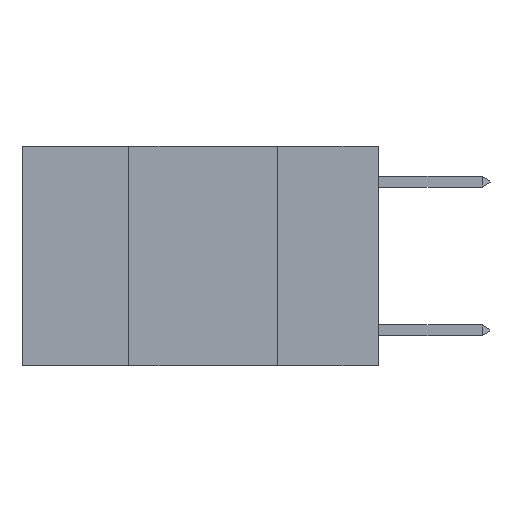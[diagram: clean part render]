
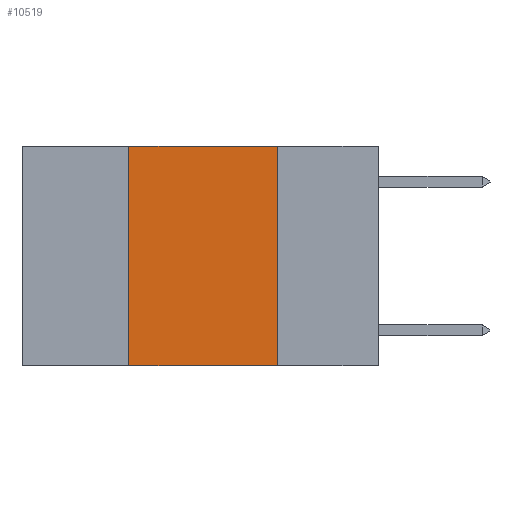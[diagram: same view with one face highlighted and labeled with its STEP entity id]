
A CAD part, left-side view. The second image highlights one B-rep face of the part: STEP entity #10519.
In plain terms, the highlighted planar face has unit normal (-1, 0, 0).
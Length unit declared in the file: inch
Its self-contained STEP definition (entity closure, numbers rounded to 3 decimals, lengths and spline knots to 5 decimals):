
#997 = EDGE_LOOP ( 'NONE', ( #5520, #3920, #13451, #10534 ) ) ;
#1403 = VECTOR ( 'NONE', #11134, 39.37008 ) ;
#1593 = LINE ( 'NONE', #3364, #11028 ) ;
#1623 = DIRECTION ( 'NONE',  ( 0., -1., 0. ) ) ;
#1652 = VECTOR ( 'NONE', #1623, 39.37008 ) ;
#2598 = CARTESIAN_POINT ( 'NONE',  ( 0., 0.17, 0. ) ) ;
#2888 = PLANE ( 'NONE',  #7925 ) ;
#3308 = CARTESIAN_POINT ( 'NONE',  ( 0., 0.17, 0. ) ) ;
#3364 = CARTESIAN_POINT ( 'NONE',  ( 0., 0.42, 0. ) ) ;
#3370 = VECTOR ( 'NONE', #3616, 39.37008 ) ;
#3616 = DIRECTION ( 'NONE',  ( 0., -1., 0. ) ) ;
#3920 = ORIENTED_EDGE ( 'NONE', *, *, #4341, .F. ) ;
#3985 = FACE_OUTER_BOUND ( 'NONE', #997, .T. ) ;
#4327 = VERTEX_POINT ( 'NONE', #8125 ) ;
#4341 = EDGE_CURVE ( 'NONE', #4327, #14167, #11317, .T. ) ;
#4520 = EDGE_CURVE ( 'NONE', #12907, #4327, #1593, .T. ) ;
#5520 = ORIENTED_EDGE ( 'NONE', *, *, #13790, .F. ) ;
#5553 = CARTESIAN_POINT ( 'NONE',  ( 0., 0.17, -0.37 ) ) ;
#7282 = CARTESIAN_POINT ( 'NONE',  ( 0., 0.6, -0.37 ) ) ;
#7313 = CARTESIAN_POINT ( 'NONE',  ( 0., 0.6, 0. ) ) ;
#7388 = CARTESIAN_POINT ( 'NONE',  ( 0., 0.42, -0.37 ) ) ;
#7925 = AXIS2_PLACEMENT_3D ( 'NONE', #7313, #11747, #8471 ) ;
#8125 = CARTESIAN_POINT ( 'NONE',  ( 0., 0.42, 0. ) ) ;
#8471 = DIRECTION ( 'NONE',  ( 0., 0., -1. ) ) ;
#9482 = DIRECTION ( 'NONE',  ( 0., 0., 1. ) ) ;
#10519 = ADVANCED_FACE ( 'NONE', ( #3985 ), #2888, .F. ) ;
#10534 = ORIENTED_EDGE ( 'NONE', *, *, #13945, .T. ) ;
#11028 = VECTOR ( 'NONE', #9482, 39.37008 ) ;
#11134 = DIRECTION ( 'NONE',  ( 0., 0., -1. ) ) ;
#11317 = LINE ( 'NONE', #13729, #3370 ) ;
#11456 = VERTEX_POINT ( 'NONE', #5553 ) ;
#11709 = LINE ( 'NONE', #7282, #1652 ) ;
#11747 = DIRECTION ( 'NONE',  ( 1., 0., 0. ) ) ;
#12249 = LINE ( 'NONE', #3308, #1403 ) ;
#12907 = VERTEX_POINT ( 'NONE', #7388 ) ;
#13451 = ORIENTED_EDGE ( 'NONE', *, *, #4520, .F. ) ;
#13729 = CARTESIAN_POINT ( 'NONE',  ( 0., 0.6, 0. ) ) ;
#13790 = EDGE_CURVE ( 'NONE', #14167, #11456, #12249, .T. ) ;
#13945 = EDGE_CURVE ( 'NONE', #12907, #11456, #11709, .T. ) ;
#14167 = VERTEX_POINT ( 'NONE', #2598 ) ;
